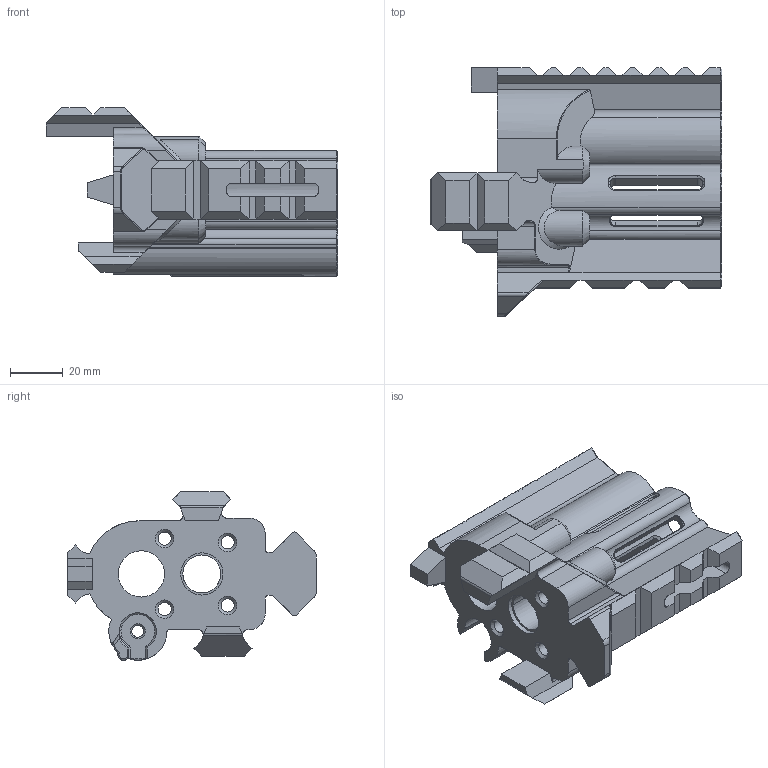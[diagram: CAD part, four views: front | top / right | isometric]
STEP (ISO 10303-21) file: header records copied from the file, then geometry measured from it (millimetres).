
FILE_DESCRIPTION(/* description */ (''),/* implementation_level */ '2;1');
FILE_NAME(/* name */ 'MOD9 V3 BARREL RETAINER.stp',/* time_stamp */ '2020-12-24T23:24:32+02:00',/* author */ (''),/* organization */ (''),/* preprocessor_version */ 'ST-DEVELOPER v15.2',/* originating_system */ 'Autodesk Translator Framework v2.0.0.5431',/* authorisation */ '');
FILE_SCHEMA (('AUTOMOTIVE_DESIGN { 1 0 10303 214 3 1 1 }'));
Length unit declared in the file: centimetre
Products named in the file (1): (Unsaved)
Bounding box: 110.59 x 94.2 x 63.85 mm (x, y, z)
Volume: 147288.4 mm3; surface area: 47553.5 mm2
Topology: 1 solids, 1 shells, 430 faces, 1116 edges, 686 vertices
Faces by surface type: plane 184, cylinder 107, bspline 76, cone 52, torus 9, sphere 2
Full cylindrical faces by diameter (mm): 4.5 x1, 5 x4, 16 x2, 17.5 x1
Entity records: 18683 total; most frequent: CARTESIAN_POINT 8678, ORIENTED_EDGE 2178, DIRECTION 1888, EDGE_CURVE 1089, VERTEX_POINT 681, AXIS2_PLACEMENT_3D 636, LINE 616, VECTOR 616
